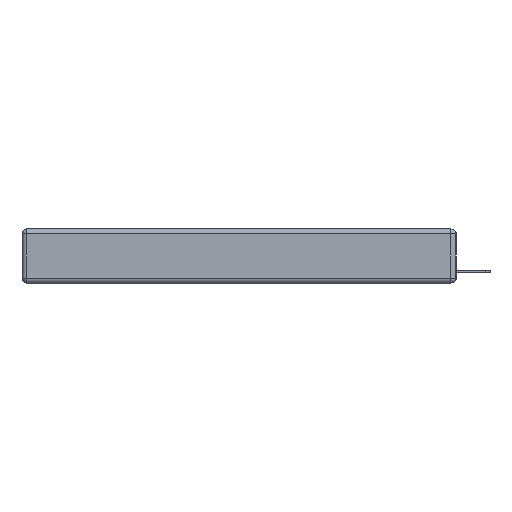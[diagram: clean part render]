
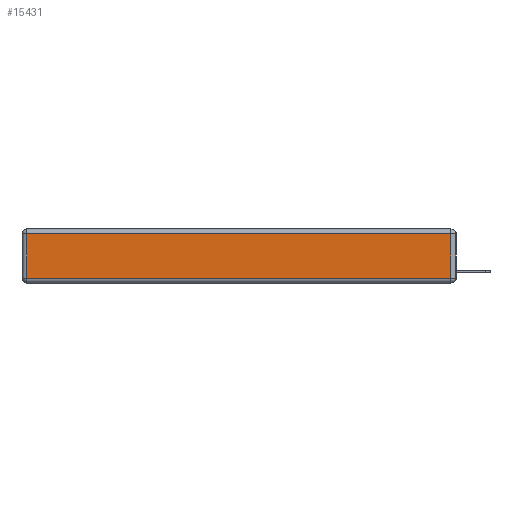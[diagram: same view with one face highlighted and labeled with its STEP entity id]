
A CAD part, left-side view. The second image highlights one B-rep face of the part: STEP entity #15431.
In plain terms, the highlighted planar face has unit normal (-1, 0, 0).
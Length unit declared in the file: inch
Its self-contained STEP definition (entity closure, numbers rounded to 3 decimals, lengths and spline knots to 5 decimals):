
#628 = VECTOR ( 'NONE', #7697, 39.37008 ) ;
#1424 = FACE_OUTER_BOUND ( 'NONE', #5120, .T. ) ;
#1682 = VERTEX_POINT ( 'NONE', #7773 ) ;
#1859 = CARTESIAN_POINT ( 'NONE',  ( 0., 2.75, -0.03 ) ) ;
#2444 = EDGE_CURVE ( 'NONE', #8950, #12389, #2681, .T. ) ;
#2681 = LINE ( 'NONE', #12843, #628 ) ;
#3677 = CARTESIAN_POINT ( 'NONE',  ( 0., 0., -0.343 ) ) ;
#3902 = EDGE_CURVE ( 'NONE', #12389, #1682, #7140, .T. ) ;
#4380 = VECTOR ( 'NONE', #11786, 39.37008 ) ;
#5120 = EDGE_LOOP ( 'NONE', ( #9525, #14437, #7343, #10745 ) ) ;
#5385 = DIRECTION ( 'NONE',  ( 0., -1., 0. ) ) ;
#7140 = LINE ( 'NONE', #12070, #13639 ) ;
#7343 = ORIENTED_EDGE ( 'NONE', *, *, #11083, .T. ) ;
#7584 = VERTEX_POINT ( 'NONE', #15540 ) ;
#7697 = DIRECTION ( 'NONE',  ( 0., 0., -1. ) ) ;
#7773 = CARTESIAN_POINT ( 'NONE',  ( 0., 0.03, -0.313 ) ) ;
#7822 = CARTESIAN_POINT ( 'NONE',  ( 0., 0.03, -0.343 ) ) ;
#7829 = LINE ( 'NONE', #7822, #4380 ) ;
#8251 = DIRECTION ( 'NONE',  ( 0., 1., 0. ) ) ;
#8950 = VERTEX_POINT ( 'NONE', #15075 ) ;
#9011 = PLANE ( 'NONE',  #12523 ) ;
#9525 = ORIENTED_EDGE ( 'NONE', *, *, #3902, .T. ) ;
#9644 = LINE ( 'NONE', #1859, #9846 ) ;
#9846 = VECTOR ( 'NONE', #8251, 39.37008 ) ;
#9992 = CARTESIAN_POINT ( 'NONE',  ( 0., 2.72, -0.313 ) ) ;
#10213 = DIRECTION ( 'NONE',  ( -1., 0., 0. ) ) ;
#10367 = EDGE_CURVE ( 'NONE', #1682, #7584, #7829, .T. ) ;
#10745 = ORIENTED_EDGE ( 'NONE', *, *, #2444, .T. ) ;
#11083 = EDGE_CURVE ( 'NONE', #7584, #8950, #9644, .T. ) ;
#11620 = DIRECTION ( 'NONE',  ( 0., 0., 1. ) ) ;
#11786 = DIRECTION ( 'NONE',  ( 0., 0., 1. ) ) ;
#12070 = CARTESIAN_POINT ( 'NONE',  ( 0., 0., -0.313 ) ) ;
#12389 = VERTEX_POINT ( 'NONE', #9992 ) ;
#12523 = AXIS2_PLACEMENT_3D ( 'NONE', #3677, #10213, #11620 ) ;
#12843 = CARTESIAN_POINT ( 'NONE',  ( 0., 2.72, -0.343 ) ) ;
#13639 = VECTOR ( 'NONE', #5385, 39.37008 ) ;
#14437 = ORIENTED_EDGE ( 'NONE', *, *, #10367, .T. ) ;
#15075 = CARTESIAN_POINT ( 'NONE',  ( 0., 2.72, -0.03 ) ) ;
#15431 = ADVANCED_FACE ( 'NONE', ( #1424 ), #9011, .T. ) ;
#15540 = CARTESIAN_POINT ( 'NONE',  ( 0., 0.03, -0.03 ) ) ;
